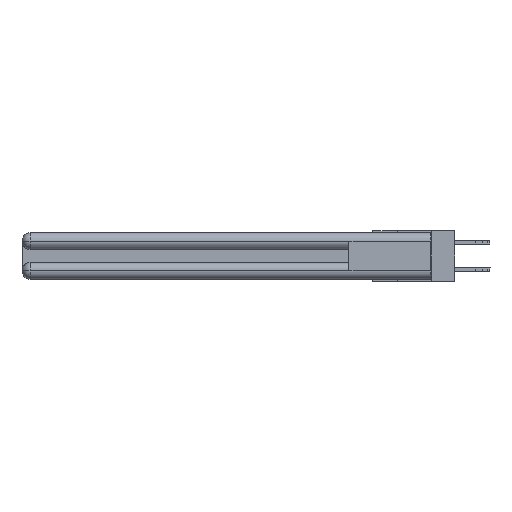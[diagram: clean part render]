
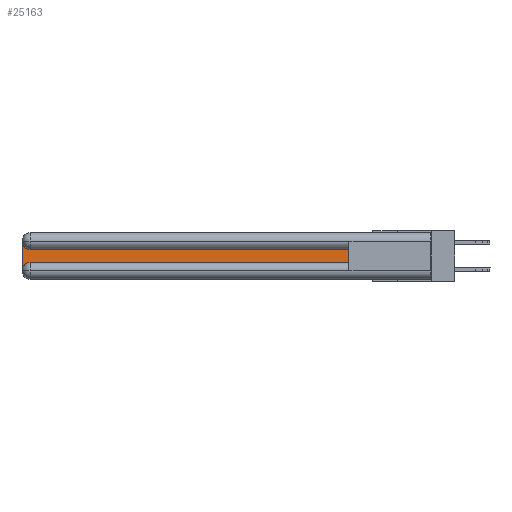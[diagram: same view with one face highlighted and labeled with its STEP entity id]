
A CAD part, left-side view. The second image highlights one B-rep face of the part: STEP entity #25163.
In plain terms, the highlighted planar face has unit normal (-1, 0, 0).
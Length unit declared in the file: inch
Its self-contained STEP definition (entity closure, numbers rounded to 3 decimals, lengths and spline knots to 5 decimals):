
#218 = ORIENTED_EDGE ( 'NONE', *, *, #18550, .T. ) ;
#322 = VERTEX_POINT ( 'NONE', #17128 ) ;
#2574 = DIRECTION ( 'NONE',  ( 1., 0., 0. ) ) ;
#3185 = VERTEX_POINT ( 'NONE', #8864 ) ;
#3344 = AXIS2_PLACEMENT_3D ( 'NONE', #7024, #2574, #23768 ) ;
#4725 = DIRECTION ( 'NONE',  ( 1., 0., 0. ) ) ;
#4754 = EDGE_CURVE ( 'NONE', #322, #15974, #11449, .T. ) ;
#4965 = DIRECTION ( 'NONE',  ( 0., 0., -1. ) ) ;
#5198 = CARTESIAN_POINT ( 'NONE',  ( 0.075, 3., -0.2175 ) ) ;
#5605 = VERTEX_POINT ( 'NONE', #9370 ) ;
#5814 = AXIS2_PLACEMENT_3D ( 'NONE', #11133, #4725, #15726 ) ;
#5896 = EDGE_CURVE ( 'NONE', #7451, #21740, #19919, .T. ) ;
#5900 = LINE ( 'NONE', #12206, #24872 ) ;
#6445 = AXIS2_PLACEMENT_3D ( 'NONE', #15618, #11208, #4965 ) ;
#6934 = CARTESIAN_POINT ( 'NONE',  ( 0.075, 0.6, -0.2175 ) ) ;
#7024 = CARTESIAN_POINT ( 'NONE',  ( 0.075, 2.94, -0.2775 ) ) ;
#7451 = VERTEX_POINT ( 'NONE', #21950 ) ;
#7827 = VECTOR ( 'NONE', #24103, 39.37008 ) ;
#8099 = VECTOR ( 'NONE', #19861, 39.37008 ) ;
#8864 = CARTESIAN_POINT ( 'NONE',  ( 0.075, 0.6, -0.1225 ) ) ;
#8870 = PLANE ( 'NONE',  #6445 ) ;
#9141 = CARTESIAN_POINT ( 'NONE',  ( 0.075, 0.6, -0.2175 ) ) ;
#9370 = CARTESIAN_POINT ( 'NONE',  ( 0.075, 3., -0.2775 ) ) ;
#9610 = FACE_OUTER_BOUND ( 'NONE', #26926, .T. ) ;
#9842 = LINE ( 'NONE', #5198, #17856 ) ;
#11133 = CARTESIAN_POINT ( 'NONE',  ( 0.075, 2.94, -0.0625 ) ) ;
#11208 = DIRECTION ( 'NONE',  ( 1., 0., 0. ) ) ;
#11449 = LINE ( 'NONE', #9141, #8099 ) ;
#12206 = CARTESIAN_POINT ( 'NONE',  ( 0.075, 0.6, -0.2175 ) ) ;
#12964 = ORIENTED_EDGE ( 'NONE', *, *, #16650, .T. ) ;
#15190 = CIRCLE ( 'NONE', #3344, 0.06 ) ;
#15618 = CARTESIAN_POINT ( 'NONE',  ( 0.075, 3., -0.1225 ) ) ;
#15726 = DIRECTION ( 'NONE',  ( 0., 0., -1. ) ) ;
#15974 = VERTEX_POINT ( 'NONE', #6934 ) ;
#16650 = EDGE_CURVE ( 'NONE', #21740, #5605, #9842, .T. ) ;
#16897 = EDGE_CURVE ( 'NONE', #5605, #322, #15190, .T. ) ;
#17128 = CARTESIAN_POINT ( 'NONE',  ( 0.075, 2.94, -0.2175 ) ) ;
#17856 = VECTOR ( 'NONE', #20208, 39.37008 ) ;
#18384 = ORIENTED_EDGE ( 'NONE', *, *, #16897, .T. ) ;
#18550 = EDGE_CURVE ( 'NONE', #3185, #7451, #27459, .T. ) ;
#19599 = CARTESIAN_POINT ( 'NONE',  ( 0.075, 3., -0.0625 ) ) ;
#19861 = DIRECTION ( 'NONE',  ( 0., -1., 0. ) ) ;
#19919 = CIRCLE ( 'NONE', #5814, 0.06 ) ;
#20208 = DIRECTION ( 'NONE',  ( 0., 0., -1. ) ) ;
#21236 = ORIENTED_EDGE ( 'NONE', *, *, #4754, .T. ) ;
#21740 = VERTEX_POINT ( 'NONE', #19599 ) ;
#21950 = CARTESIAN_POINT ( 'NONE',  ( 0.075, 2.94, -0.1225 ) ) ;
#22257 = ORIENTED_EDGE ( 'NONE', *, *, #26229, .T. ) ;
#23768 = DIRECTION ( 'NONE',  ( 0., 0., -1. ) ) ;
#24103 = DIRECTION ( 'NONE',  ( 0., 1., 0. ) ) ;
#24872 = VECTOR ( 'NONE', #26975, 39.37008 ) ;
#25137 = ORIENTED_EDGE ( 'NONE', *, *, #5896, .T. ) ;
#25163 = ADVANCED_FACE ( 'NONE', ( #9610 ), #8870, .F. ) ;
#26229 = EDGE_CURVE ( 'NONE', #15974, #3185, #5900, .T. ) ;
#26260 = CARTESIAN_POINT ( 'NONE',  ( 0.075, 0.6, -0.1225 ) ) ;
#26926 = EDGE_LOOP ( 'NONE', ( #218, #25137, #12964, #18384, #21236, #22257 ) ) ;
#26975 = DIRECTION ( 'NONE',  ( 0., 0., 1. ) ) ;
#27459 = LINE ( 'NONE', #26260, #7827 ) ;
